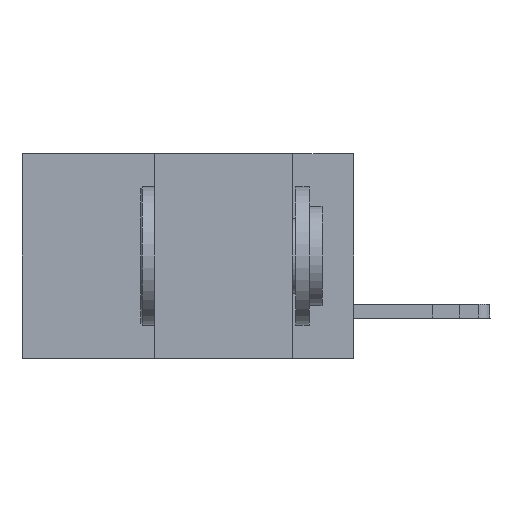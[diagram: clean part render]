
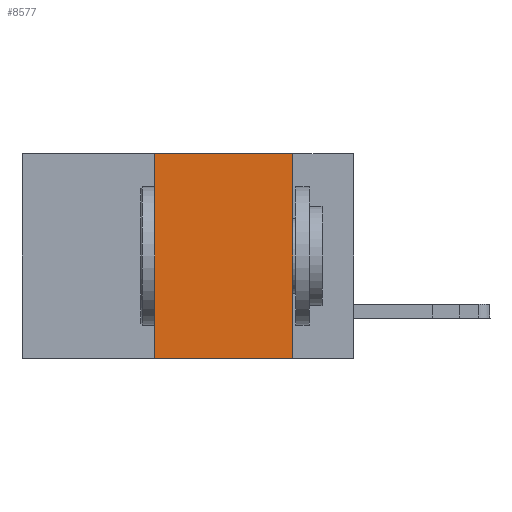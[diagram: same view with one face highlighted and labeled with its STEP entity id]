
A CAD part, left-side view. The second image highlights one B-rep face of the part: STEP entity #8577.
In plain terms, the highlighted planar face has unit normal (-1, 0, 0).
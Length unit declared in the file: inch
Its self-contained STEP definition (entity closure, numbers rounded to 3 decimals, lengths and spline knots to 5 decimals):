
#2417 = VECTOR ( 'NONE', #3928, 39.37008 ) ;
#3638 = DIRECTION ( 'NONE',  ( 0., 0., -1. ) ) ;
#3928 = DIRECTION ( 'NONE',  ( 0., 0., 1. ) ) ;
#5841 = VECTOR ( 'NONE', #10693, 39.37008 ) ;
#6253 = VERTEX_POINT ( 'NONE', #7882 ) ;
#7333 = EDGE_CURVE ( 'NONE', #7820, #9273, #11908, .T. ) ;
#7346 = CARTESIAN_POINT ( 'NONE',  ( 0., 0.36, 0. ) ) ;
#7686 = LINE ( 'NONE', #12317, #5841 ) ;
#7701 = CARTESIAN_POINT ( 'NONE',  ( 0., 0.11, -0.37 ) ) ;
#7820 = VERTEX_POINT ( 'NONE', #8544 ) ;
#7882 = CARTESIAN_POINT ( 'NONE',  ( 0., 0.36, 0. ) ) ;
#8544 = CARTESIAN_POINT ( 'NONE',  ( 0., 0.11, 0. ) ) ;
#8577 = ADVANCED_FACE ( 'NONE', ( #9672 ), #17841, .F. ) ;
#8607 = ORIENTED_EDGE ( 'NONE', *, *, #7333, .F. ) ;
#9273 = VERTEX_POINT ( 'NONE', #7701 ) ;
#9672 = FACE_OUTER_BOUND ( 'NONE', #11238, .T. ) ;
#10529 = ORIENTED_EDGE ( 'NONE', *, *, #18840, .T. ) ;
#10693 = DIRECTION ( 'NONE',  ( 0., -1., 0. ) ) ;
#11238 = EDGE_LOOP ( 'NONE', ( #8607, #11907, #13236, #10529 ) ) ;
#11292 = CARTESIAN_POINT ( 'NONE',  ( 0., 0.6, 0. ) ) ;
#11759 = LINE ( 'NONE', #7346, #2417 ) ;
#11788 = AXIS2_PLACEMENT_3D ( 'NONE', #19853, #16326, #14822 ) ;
#11907 = ORIENTED_EDGE ( 'NONE', *, *, #17473, .F. ) ;
#11908 = LINE ( 'NONE', #13834, #20751 ) ;
#12317 = CARTESIAN_POINT ( 'NONE',  ( 0., 0.6, -0.37 ) ) ;
#12425 = VERTEX_POINT ( 'NONE', #19104 ) ;
#13236 = ORIENTED_EDGE ( 'NONE', *, *, #20293, .F. ) ;
#13834 = CARTESIAN_POINT ( 'NONE',  ( 0., 0.11, 0. ) ) ;
#14411 = LINE ( 'NONE', #11292, #19844 ) ;
#14623 = DIRECTION ( 'NONE',  ( 0., -1., 0. ) ) ;
#14822 = DIRECTION ( 'NONE',  ( 0., 0., -1. ) ) ;
#16326 = DIRECTION ( 'NONE',  ( 1., 0., 0. ) ) ;
#17473 = EDGE_CURVE ( 'NONE', #6253, #7820, #14411, .T. ) ;
#17841 = PLANE ( 'NONE',  #11788 ) ;
#18840 = EDGE_CURVE ( 'NONE', #12425, #9273, #7686, .T. ) ;
#19104 = CARTESIAN_POINT ( 'NONE',  ( 0., 0.36, -0.37 ) ) ;
#19844 = VECTOR ( 'NONE', #14623, 39.37008 ) ;
#19853 = CARTESIAN_POINT ( 'NONE',  ( 0., 0.6, 0. ) ) ;
#20293 = EDGE_CURVE ( 'NONE', #12425, #6253, #11759, .T. ) ;
#20751 = VECTOR ( 'NONE', #3638, 39.37008 ) ;
